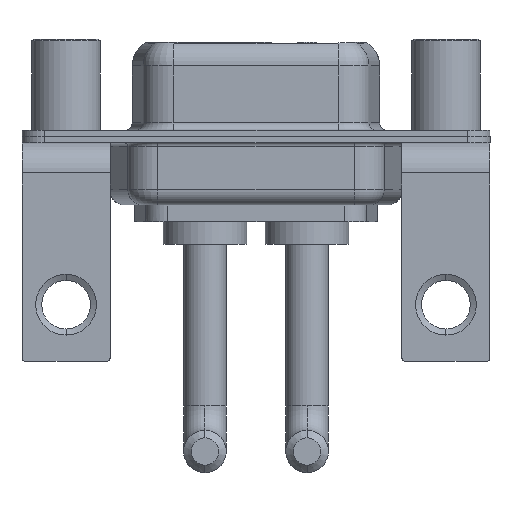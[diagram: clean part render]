
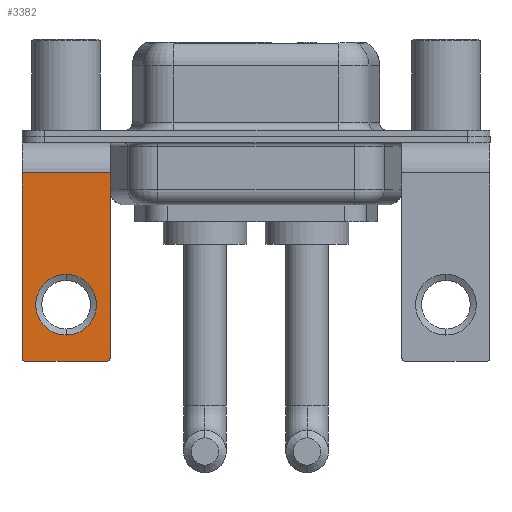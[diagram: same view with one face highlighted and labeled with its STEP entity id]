
A CAD part, front view. The second image highlights one B-rep face of the part: STEP entity #3382.
In plain terms, the highlighted planar face has unit normal (0, -1, 0).
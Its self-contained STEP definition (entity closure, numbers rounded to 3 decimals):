
#164 = AXIS2_PLACEMENT_3D ( 'NONE', #5387, #10288, #9065 ) ;
#1085 = DIRECTION ( 'NONE',  ( 0., 1., 0. ) ) ;
#1374 = FACE_OUTER_BOUND ( 'NONE', #3322, .T. ) ;
#1391 = CARTESIAN_POINT ( 'NONE',  ( 0., -6.25, -11.07 ) ) ;
#1473 = VERTEX_POINT ( 'NONE', #9189 ) ;
#1650 = EDGE_CURVE ( 'NONE', #11650, #2256, #2532, .T. ) ;
#1757 = CIRCLE ( 'NONE', #12289, 0.25 ) ;
#2256 = VERTEX_POINT ( 'NONE', #8737 ) ;
#2269 = CARTESIAN_POINT ( 'NONE',  ( 2.9, -6.25, -2.4 ) ) ;
#2321 = EDGE_CURVE ( 'NONE', #9244, #3011, #9279, .T. ) ;
#2421 = DIRECTION ( 'NONE',  ( -1., 0., 0. ) ) ;
#2532 = CIRCLE ( 'NONE', #13825, 2. ) ;
#2569 = PLANE ( 'NONE',  #9743 ) ;
#2726 = ORIENTED_EDGE ( 'NONE', *, *, #8521, .T. ) ;
#2727 = FACE_BOUND ( 'NONE', #15462, .T. ) ;
#2813 = CARTESIAN_POINT ( 'NONE',  ( 2.9, -6.25, -2.4 ) ) ;
#3011 = VERTEX_POINT ( 'NONE', #10058 ) ;
#3040 = DIRECTION ( 'NONE',  ( 0., 0., 1. ) ) ;
#3168 = CARTESIAN_POINT ( 'NONE',  ( 2.9, -6.25, -2.4 ) ) ;
#3322 = EDGE_LOOP ( 'NONE', ( #5626, #6882, #11163, #14429, #4647, #13101 ) ) ;
#3323 = CARTESIAN_POINT ( 'NONE',  ( 2.9, -6.25, -2.4 ) ) ;
#3382 = ADVANCED_FACE ( 'NONE', ( #2727, #1374 ), #2569, .F. ) ;
#3547 = CARTESIAN_POINT ( 'NONE',  ( -2.65, -6.25, -14.8 ) ) ;
#3595 = DIRECTION ( 'NONE',  ( 0., 0., 1. ) ) ;
#4238 = VECTOR ( 'NONE', #8221, 1000. ) ;
#4642 = CARTESIAN_POINT ( 'NONE',  ( 0., -6.25, -11.07 ) ) ;
#4647 = ORIENTED_EDGE ( 'NONE', *, *, #9686, .F. ) ;
#4980 = EDGE_CURVE ( 'NONE', #9579, #1473, #12469, .T. ) ;
#5387 = CARTESIAN_POINT ( 'NONE',  ( 2.65, -6.25, -14.55 ) ) ;
#5413 = DIRECTION ( 'NONE',  ( 0., -1., 0. ) ) ;
#5626 = ORIENTED_EDGE ( 'NONE', *, *, #2321, .T. ) ;
#6093 = CARTESIAN_POINT ( 'NONE',  ( 2.9, -6.25, -14.8 ) ) ;
#6287 = DIRECTION ( 'NONE',  ( 0., 0., 1. ) ) ;
#6425 = DIRECTION ( 'NONE',  ( 0., 1., 0. ) ) ;
#6512 = AXIS2_PLACEMENT_3D ( 'NONE', #4642, #15305, #3040 ) ;
#6882 = ORIENTED_EDGE ( 'NONE', *, *, #12787, .T. ) ;
#7171 = LINE ( 'NONE', #2269, #12461 ) ;
#7529 = VECTOR ( 'NONE', #13392, 1000. ) ;
#7684 = EDGE_CURVE ( 'NONE', #9579, #13973, #9614, .T. ) ;
#7798 = CIRCLE ( 'NONE', #6512, 2. ) ;
#7979 = VERTEX_POINT ( 'NONE', #3168 ) ;
#8221 = DIRECTION ( 'NONE',  ( 0., 0., -1. ) ) ;
#8464 = LINE ( 'NONE', #3323, #4238 ) ;
#8521 = EDGE_CURVE ( 'NONE', #2256, #11650, #7798, .T. ) ;
#8737 = CARTESIAN_POINT ( 'NONE',  ( 0., -6.25, -9.07 ) ) ;
#9065 = DIRECTION ( 'NONE',  ( 0., 0., 1. ) ) ;
#9189 = CARTESIAN_POINT ( 'NONE',  ( 2.9, -6.25, -14.55 ) ) ;
#9244 = VERTEX_POINT ( 'NONE', #9917 ) ;
#9279 = LINE ( 'NONE', #15209, #11872 ) ;
#9579 = VERTEX_POINT ( 'NONE', #14465 ) ;
#9614 = LINE ( 'NONE', #6093, #7529 ) ;
#9686 = EDGE_CURVE ( 'NONE', #7979, #1473, #8464, .T. ) ;
#9743 = AXIS2_PLACEMENT_3D ( 'NONE', #2813, #6425, #10203 ) ;
#9859 = ORIENTED_EDGE ( 'NONE', *, *, #1650, .T. ) ;
#9917 = CARTESIAN_POINT ( 'NONE',  ( -2.9, -6.25, -2.4 ) ) ;
#10058 = CARTESIAN_POINT ( 'NONE',  ( -2.9, -6.25, -14.55 ) ) ;
#10203 = DIRECTION ( 'NONE',  ( 0., 0., 1. ) ) ;
#10288 = DIRECTION ( 'NONE',  ( 0., -1., 0. ) ) ;
#11163 = ORIENTED_EDGE ( 'NONE', *, *, #7684, .F. ) ;
#11650 = VERTEX_POINT ( 'NONE', #13184 ) ;
#11872 = VECTOR ( 'NONE', #15143, 1000. ) ;
#12289 = AXIS2_PLACEMENT_3D ( 'NONE', #12732, #5413, #3595 ) ;
#12461 = VECTOR ( 'NONE', #2421, 1000. ) ;
#12469 = CIRCLE ( 'NONE', #164, 0.25 ) ;
#12732 = CARTESIAN_POINT ( 'NONE',  ( -2.65, -6.25, -14.55 ) ) ;
#12787 = EDGE_CURVE ( 'NONE', #3011, #13973, #1757, .T. ) ;
#13101 = ORIENTED_EDGE ( 'NONE', *, *, #15455, .T. ) ;
#13184 = CARTESIAN_POINT ( 'NONE',  ( 0., -6.25, -13.07 ) ) ;
#13392 = DIRECTION ( 'NONE',  ( -1., 0., 0. ) ) ;
#13825 = AXIS2_PLACEMENT_3D ( 'NONE', #1391, #1085, #6287 ) ;
#13973 = VERTEX_POINT ( 'NONE', #3547 ) ;
#14429 = ORIENTED_EDGE ( 'NONE', *, *, #4980, .T. ) ;
#14465 = CARTESIAN_POINT ( 'NONE',  ( 2.65, -6.25, -14.8 ) ) ;
#15143 = DIRECTION ( 'NONE',  ( 0., 0., -1. ) ) ;
#15209 = CARTESIAN_POINT ( 'NONE',  ( -2.9, -6.25, -2.4 ) ) ;
#15305 = DIRECTION ( 'NONE',  ( 0., 1., 0. ) ) ;
#15455 = EDGE_CURVE ( 'NONE', #7979, #9244, #7171, .T. ) ;
#15462 = EDGE_LOOP ( 'NONE', ( #9859, #2726 ) ) ;
